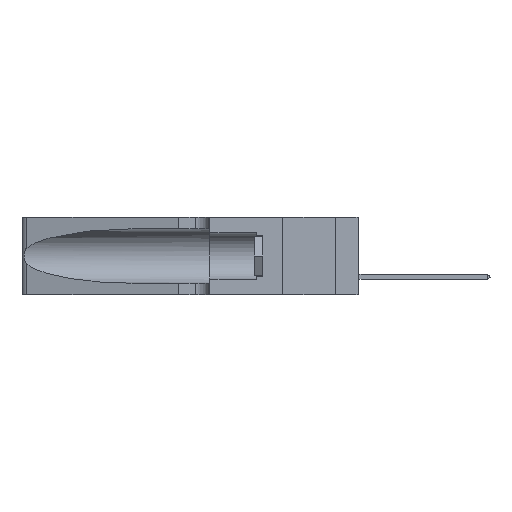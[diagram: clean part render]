
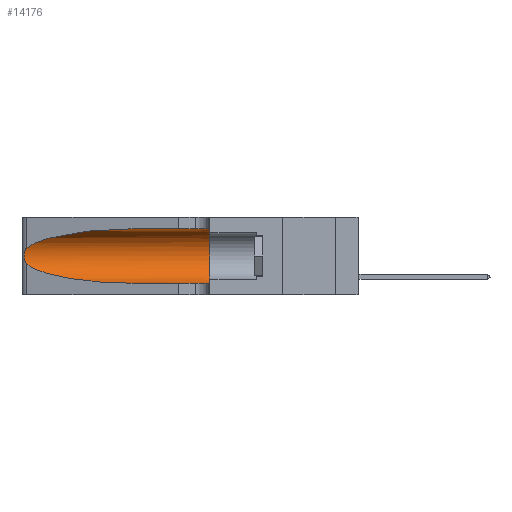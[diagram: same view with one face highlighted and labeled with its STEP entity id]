
A CAD part, left-side view. The second image highlights one B-rep face of the part: STEP entity #14176.
In plain terms, the highlighted cylindrical face has radius 3.308 mm (diameter 6.617 mm), a partial arc.
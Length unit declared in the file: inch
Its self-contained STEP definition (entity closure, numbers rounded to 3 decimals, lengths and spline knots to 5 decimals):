
#223 = CARTESIAN_POINT ( 'NONE',  ( 0.26075, 1.23896, 0.19203 ) ) ;
#973 = CARTESIAN_POINT ( 'NONE',  ( 0.1305, 1.61858, 0.05475 ) ) ;
#1015 = CARTESIAN_POINT ( 'NONE',  ( 0.2373, 1.15595, 0.08982 ) ) ;
#1161 = CARTESIAN_POINT ( 'NONE',  ( 0.18966, 0.96281, 0.05475 ) ) ;
#1331 = CARTESIAN_POINT ( 'NONE',  ( 0.1305, 0.72297, 0.31525 ) ) ;
#1823 =( BOUNDED_CURVE ( )  B_SPLINE_CURVE ( 3, ( #7516, #17481, #7378, #20932 ),
 .UNSPECIFIED., .F., .F. ) 
 B_SPLINE_CURVE_WITH_KNOTS ( ( 4, 4 ),
 ( 1.5708, 2.84003 ),
 .UNSPECIFIED. ) 
 CURVE ( )  GEOMETRIC_REPRESENTATION_ITEM ( )  RATIONAL_B_SPLINE_CURVE ( ( 1., 0.87, 0.87, 1. ) ) 
 REPRESENTATION_ITEM ( '' )  );
#2078 = VERTEX_POINT ( 'NONE', #9839 ) ;
#2099 = CARTESIAN_POINT ( 'NONE',  ( 0.25487, 1.22718, 0.14631 ) ) ;
#2464 = CARTESIAN_POINT ( 'NONE',  ( 0.1305, 0.72297, 0.05475 ) ) ;
#2803 = ORIENTED_EDGE ( 'NONE', *, *, #15194, .T. ) ;
#3581 = ORIENTED_EDGE ( 'NONE', *, *, #6041, .T. ) ;
#4206 = EDGE_LOOP ( 'NONE', ( #17523, #3581, #2803, #21311, #20033, #11090 ) ) ;
#4691 = CARTESIAN_POINT ( 'NONE',  ( 0.1305, 1.61858, 0.185 ) ) ;
#5005 = CARTESIAN_POINT ( 'NONE',  ( 0.25854, 1.2359, 0.20912 ) ) ;
#5222 = CARTESIAN_POINT ( 'NONE',  ( 0.26018, 1.23835, 0.19895 ) ) ;
#5298 = CARTESIAN_POINT ( 'NONE',  ( 0.25555, 1.22993, 0.14849 ) ) ;
#5999 = B_SPLINE_CURVE_WITH_KNOTS ( 'NONE', 3,
 ( #15140, #6682, #19930, #11921, #5005, #5222, #223, #6757, #9998, #13587, #20010, #15202, #5298, #16853 ),
 .UNSPECIFIED., .F., .F.,
 ( 4, 2, 2, 2, 2, 2, 4 ),
 ( 0., 0.00027, 0.00053, 0.00107, 0.0016, 0.00187, 0.00214 ),
 .UNSPECIFIED. ) ;
#6041 = EDGE_CURVE ( 'NONE', #18802, #14911, #5999, .T. ) ;
#6336 = DIRECTION ( 'NONE',  ( 0., -1., 0. ) ) ;
#6653 = EDGE_CURVE ( 'NONE', #11888, #13829, #17056, .T. ) ;
#6682 = CARTESIAN_POINT ( 'NONE',  ( 0.25555, 1.22994, 0.2215 ) ) ;
#6757 = CARTESIAN_POINT ( 'NONE',  ( 0.26075, 1.23896, 0.178 ) ) ;
#6855 = EDGE_CURVE ( 'NONE', #2078, #13829, #14030, .T. ) ;
#7378 = CARTESIAN_POINT ( 'NONE',  ( 0.2373, 1.15595, 0.28018 ) ) ;
#7516 = CARTESIAN_POINT ( 'NONE',  ( 0.1305, 0.72297, 0.31525 ) ) ;
#7655 = CARTESIAN_POINT ( 'NONE',  ( 0.1305, 0.35, 0.185 ) ) ;
#9142 = CARTESIAN_POINT ( 'NONE',  ( 0.1305, 0.35, 0.05475 ) ) ;
#9389 = DIRECTION ( 'NONE',  ( 0., -1., 0. ) ) ;
#9764 = EDGE_CURVE ( 'NONE', #20275, #18802, #1823, .T. ) ;
#9839 = CARTESIAN_POINT ( 'NONE',  ( 0.1305, 0.35, 0.31525 ) ) ;
#9917 = LINE ( 'NONE', #21211, #11788 ) ;
#9998 = CARTESIAN_POINT ( 'NONE',  ( 0.26017, 1.23833, 0.17102 ) ) ;
#10353 =( BOUNDED_CURVE ( )  B_SPLINE_CURVE ( 3, ( #11094, #1015, #1161, #2464 ),
 .UNSPECIFIED., .F., .T. ) 
 B_SPLINE_CURVE_WITH_KNOTS ( ( 4, 4 ),
 ( 3.44316, 4.71239 ),
 .UNSPECIFIED. ) 
 CURVE ( )  GEOMETRIC_REPRESENTATION_ITEM ( )  RATIONAL_B_SPLINE_CURVE ( ( 1., 0.87, 0.87, 1. ) ) 
 REPRESENTATION_ITEM ( '' )  );
#10829 = AXIS2_PLACEMENT_3D ( 'NONE', #7655, #17323, #12621 ) ;
#11090 = ORIENTED_EDGE ( 'NONE', *, *, #13193, .F. ) ;
#11094 = CARTESIAN_POINT ( 'NONE',  ( 0.25487, 1.22718, 0.14631 ) ) ;
#11788 = VECTOR ( 'NONE', #6336, 39.37008 ) ;
#11888 = VERTEX_POINT ( 'NONE', #15480 ) ;
#11921 = CARTESIAN_POINT ( 'NONE',  ( 0.25787, 1.23484, 0.2124 ) ) ;
#11974 = DIRECTION ( 'NONE',  ( 0., -1., 0. ) ) ;
#12621 = DIRECTION ( 'NONE',  ( 0., 0., 1. ) ) ;
#13193 = EDGE_CURVE ( 'NONE', #20275, #2078, #9917, .T. ) ;
#13587 = CARTESIAN_POINT ( 'NONE',  ( 0.25856, 1.23593, 0.16098 ) ) ;
#13706 = DIRECTION ( 'NONE',  ( 0., 0., -1. ) ) ;
#13829 = VERTEX_POINT ( 'NONE', #9142 ) ;
#14030 = CIRCLE ( 'NONE', #10829, 0.13025 ) ;
#14176 = ADVANCED_FACE ( 'NONE', ( #19440 ), #18643, .F. ) ;
#14911 = VERTEX_POINT ( 'NONE', #2099 ) ;
#15140 = CARTESIAN_POINT ( 'NONE',  ( 0.25487, 1.22718, 0.22369 ) ) ;
#15194 = EDGE_CURVE ( 'NONE', #14911, #11888, #10353, .T. ) ;
#15202 = CARTESIAN_POINT ( 'NONE',  ( 0.25639, 1.23186, 0.15144 ) ) ;
#15271 = VECTOR ( 'NONE', #9389, 39.37008 ) ;
#15480 = CARTESIAN_POINT ( 'NONE',  ( 0.1305, 0.72297, 0.05475 ) ) ;
#16463 = AXIS2_PLACEMENT_3D ( 'NONE', #4691, #11974, #13706 ) ;
#16853 = CARTESIAN_POINT ( 'NONE',  ( 0.25487, 1.22718, 0.14631 ) ) ;
#17056 = LINE ( 'NONE', #973, #15271 ) ;
#17323 = DIRECTION ( 'NONE',  ( 0., 1., 0. ) ) ;
#17481 = CARTESIAN_POINT ( 'NONE',  ( 0.18966, 0.96281, 0.31525 ) ) ;
#17523 = ORIENTED_EDGE ( 'NONE', *, *, #9764, .T. ) ;
#18643 = CYLINDRICAL_SURFACE ( 'NONE', #16463, 0.13025 ) ;
#18802 = VERTEX_POINT ( 'NONE', #19306 ) ;
#19306 = CARTESIAN_POINT ( 'NONE',  ( 0.25487, 1.22718, 0.22369 ) ) ;
#19440 = FACE_OUTER_BOUND ( 'NONE', #4206, .T. ) ;
#19930 = CARTESIAN_POINT ( 'NONE',  ( 0.25639, 1.23184, 0.21858 ) ) ;
#20010 = CARTESIAN_POINT ( 'NONE',  ( 0.25789, 1.23486, 0.15765 ) ) ;
#20033 = ORIENTED_EDGE ( 'NONE', *, *, #6855, .F. ) ;
#20275 = VERTEX_POINT ( 'NONE', #1331 ) ;
#20932 = CARTESIAN_POINT ( 'NONE',  ( 0.25487, 1.22718, 0.22369 ) ) ;
#21211 = CARTESIAN_POINT ( 'NONE',  ( 0.1305, 1.61858, 0.31525 ) ) ;
#21311 = ORIENTED_EDGE ( 'NONE', *, *, #6653, .T. ) ;
